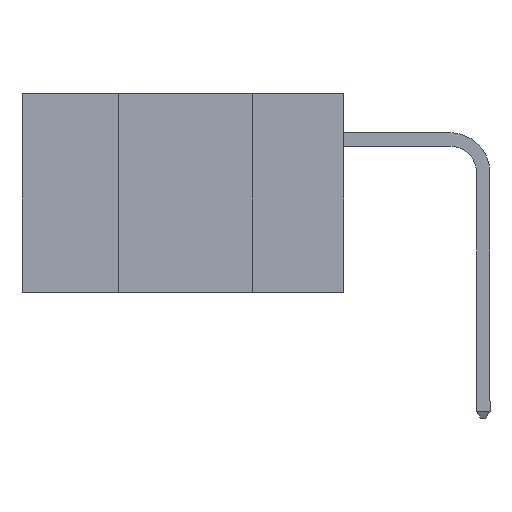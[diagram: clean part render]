
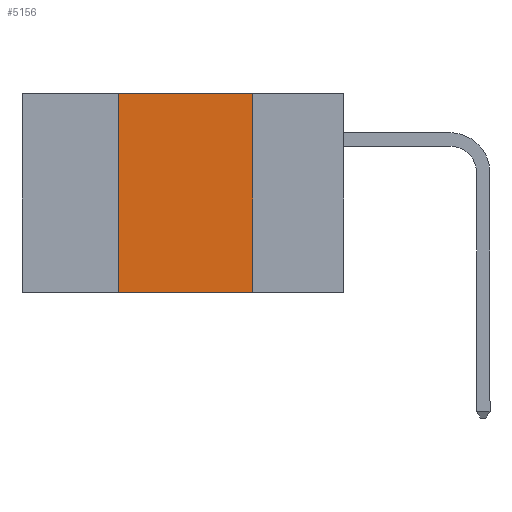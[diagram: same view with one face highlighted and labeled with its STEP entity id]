
A CAD part, left-side view. The second image highlights one B-rep face of the part: STEP entity #5156.
In plain terms, the highlighted planar face has unit normal (-1, 0, 0).
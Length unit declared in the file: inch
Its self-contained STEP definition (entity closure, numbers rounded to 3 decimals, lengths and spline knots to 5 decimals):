
#206 = LINE ( 'NONE', #9247, #8094 ) ;
#326 = CARTESIAN_POINT ( 'NONE',  ( 0., 0.6, 0. ) ) ;
#438 = VECTOR ( 'NONE', #923, 39.37008 ) ;
#923 = DIRECTION ( 'NONE',  ( 0., 0., 1. ) ) ;
#1125 = LINE ( 'NONE', #7490, #6733 ) ;
#1161 = DIRECTION ( 'NONE',  ( 1., 0., 0. ) ) ;
#1250 = VERTEX_POINT ( 'NONE', #5776 ) ;
#1627 = EDGE_CURVE ( 'NONE', #1250, #8006, #4134, .T. ) ;
#2638 = CARTESIAN_POINT ( 'NONE',  ( 0., 0.42, -0.37 ) ) ;
#2803 = ORIENTED_EDGE ( 'NONE', *, *, #7680, .F. ) ;
#3055 = VERTEX_POINT ( 'NONE', #6877 ) ;
#3213 = LINE ( 'NONE', #9087, #9276 ) ;
#3214 = ORIENTED_EDGE ( 'NONE', *, *, #6696, .F. ) ;
#3432 = ORIENTED_EDGE ( 'NONE', *, *, #1627, .F. ) ;
#3808 = DIRECTION ( 'NONE',  ( 0., -1., 0. ) ) ;
#4134 = LINE ( 'NONE', #2638, #438 ) ;
#4207 = CARTESIAN_POINT ( 'NONE',  ( 0., 0.17, 0. ) ) ;
#4394 = EDGE_LOOP ( 'NONE', ( #2803, #3214, #3432, #4581 ) ) ;
#4415 = CARTESIAN_POINT ( 'NONE',  ( 0., 0.42, 0. ) ) ;
#4581 = ORIENTED_EDGE ( 'NONE', *, *, #6395, .T. ) ;
#4711 = DIRECTION ( 'NONE',  ( 0., 0., -1. ) ) ;
#5156 = ADVANCED_FACE ( 'NONE', ( #6989 ), #9344, .F. ) ;
#5650 = DIRECTION ( 'NONE',  ( 0., -1., 0. ) ) ;
#5776 = CARTESIAN_POINT ( 'NONE',  ( 0., 0.42, -0.37 ) ) ;
#5835 = AXIS2_PLACEMENT_3D ( 'NONE', #326, #1161, #6502 ) ;
#6395 = EDGE_CURVE ( 'NONE', #1250, #3055, #1125, .T. ) ;
#6502 = DIRECTION ( 'NONE',  ( 0., 0., -1. ) ) ;
#6696 = EDGE_CURVE ( 'NONE', #8006, #8326, #206, .T. ) ;
#6733 = VECTOR ( 'NONE', #3808, 39.37008 ) ;
#6877 = CARTESIAN_POINT ( 'NONE',  ( 0., 0.17, -0.37 ) ) ;
#6989 = FACE_OUTER_BOUND ( 'NONE', #4394, .T. ) ;
#7490 = CARTESIAN_POINT ( 'NONE',  ( 0., 0.6, -0.37 ) ) ;
#7680 = EDGE_CURVE ( 'NONE', #8326, #3055, #3213, .T. ) ;
#8006 = VERTEX_POINT ( 'NONE', #4415 ) ;
#8094 = VECTOR ( 'NONE', #5650, 39.37008 ) ;
#8326 = VERTEX_POINT ( 'NONE', #4207 ) ;
#9087 = CARTESIAN_POINT ( 'NONE',  ( 0., 0.17, -0.37 ) ) ;
#9247 = CARTESIAN_POINT ( 'NONE',  ( 0., 0.6, 0. ) ) ;
#9276 = VECTOR ( 'NONE', #4711, 39.37008 ) ;
#9344 = PLANE ( 'NONE',  #5835 ) ;
